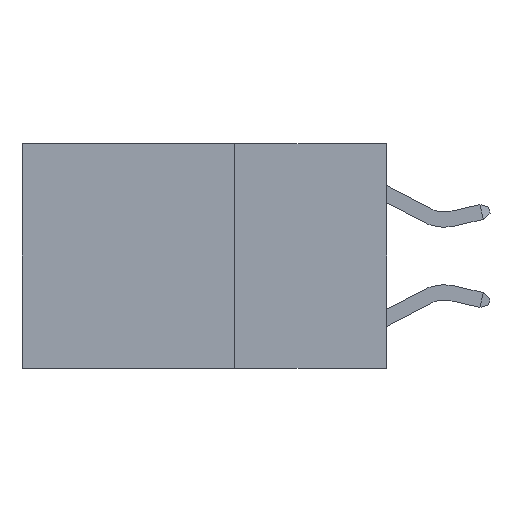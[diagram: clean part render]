
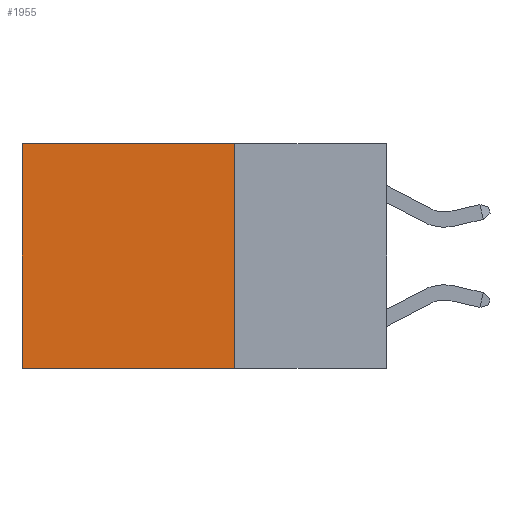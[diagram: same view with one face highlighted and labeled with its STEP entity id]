
A CAD part, left-side view. The second image highlights one B-rep face of the part: STEP entity #1955.
In plain terms, the highlighted planar face has unit normal (-1, 0, 0).
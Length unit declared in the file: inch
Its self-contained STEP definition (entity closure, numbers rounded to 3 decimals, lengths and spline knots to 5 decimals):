
#797 = CARTESIAN_POINT ( 'NONE',  ( 0.2625, 0.25, 0. ) ) ;
#1557 = LINE ( 'NONE', #10669, #12563 ) ;
#1955 = ADVANCED_FACE ( 'NONE', ( #2693 ), #10792, .F. ) ;
#2214 = DIRECTION ( 'NONE',  ( 0., 0., -1. ) ) ;
#2307 = LINE ( 'NONE', #10646, #10351 ) ;
#2693 = FACE_OUTER_BOUND ( 'NONE', #12139, .T. ) ;
#2970 = VERTEX_POINT ( 'NONE', #10345 ) ;
#3210 = EDGE_CURVE ( 'NONE', #10839, #3514, #1557, .T. ) ;
#3400 = ORIENTED_EDGE ( 'NONE', *, *, #3601, .T. ) ;
#3514 = VERTEX_POINT ( 'NONE', #11148 ) ;
#3601 = EDGE_CURVE ( 'NONE', #2970, #3514, #7116, .T. ) ;
#4301 = ORIENTED_EDGE ( 'NONE', *, *, #3210, .F. ) ;
#4610 = DIRECTION ( 'NONE',  ( 0., 0., -1. ) ) ;
#4643 = DIRECTION ( 'NONE',  ( 0., 1., 0. ) ) ;
#4767 = CARTESIAN_POINT ( 'NONE',  ( 0.2625, 0.25, 0. ) ) ;
#4856 = AXIS2_PLACEMENT_3D ( 'NONE', #4767, #5790, #12773 ) ;
#5103 = LINE ( 'NONE', #5660, #9797 ) ;
#5660 = CARTESIAN_POINT ( 'NONE',  ( 0.2625, 0.25, 0. ) ) ;
#5790 = DIRECTION ( 'NONE',  ( 1., 0., 0. ) ) ;
#6300 = CARTESIAN_POINT ( 'NONE',  ( 0.2625, 0.6, 0. ) ) ;
#7116 = LINE ( 'NONE', #6300, #9891 ) ;
#7471 = CARTESIAN_POINT ( 'NONE',  ( 0.2625, 0.25, -0.37 ) ) ;
#8455 = EDGE_CURVE ( 'NONE', #12250, #10839, #2307, .T. ) ;
#9649 = ORIENTED_EDGE ( 'NONE', *, *, #8455, .F. ) ;
#9797 = VECTOR ( 'NONE', #11665, 39.37008 ) ;
#9891 = VECTOR ( 'NONE', #2214, 39.37008 ) ;
#10345 = CARTESIAN_POINT ( 'NONE',  ( 0.2625, 0.6, 0. ) ) ;
#10351 = VECTOR ( 'NONE', #4610, 39.37008 ) ;
#10369 = EDGE_CURVE ( 'NONE', #12250, #2970, #5103, .T. ) ;
#10646 = CARTESIAN_POINT ( 'NONE',  ( 0.2625, 0.25, 0. ) ) ;
#10669 = CARTESIAN_POINT ( 'NONE',  ( 0.2625, 0.25, -0.37 ) ) ;
#10792 = PLANE ( 'NONE',  #4856 ) ;
#10839 = VERTEX_POINT ( 'NONE', #7471 ) ;
#11148 = CARTESIAN_POINT ( 'NONE',  ( 0.2625, 0.6, -0.37 ) ) ;
#11665 = DIRECTION ( 'NONE',  ( 0., 1., 0. ) ) ;
#12139 = EDGE_LOOP ( 'NONE', ( #3400, #4301, #9649, #12832 ) ) ;
#12250 = VERTEX_POINT ( 'NONE', #797 ) ;
#12563 = VECTOR ( 'NONE', #4643, 39.37008 ) ;
#12773 = DIRECTION ( 'NONE',  ( 0., 0., -1. ) ) ;
#12832 = ORIENTED_EDGE ( 'NONE', *, *, #10369, .T. ) ;
